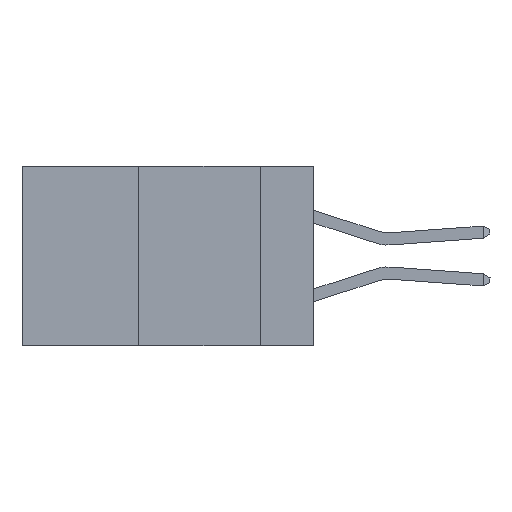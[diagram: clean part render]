
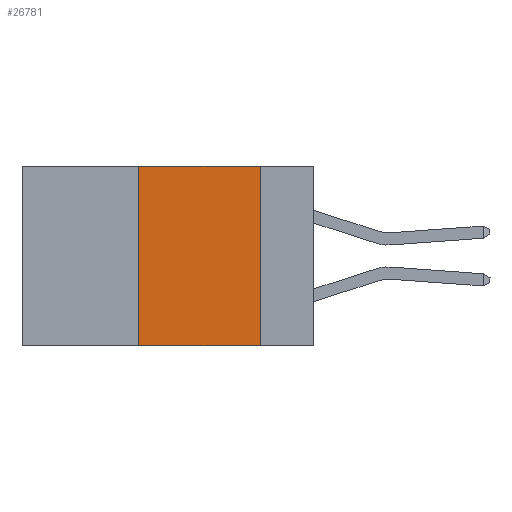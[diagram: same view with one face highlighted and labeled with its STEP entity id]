
A CAD part, left-side view. The second image highlights one B-rep face of the part: STEP entity #26781.
In plain terms, the highlighted planar face has unit normal (-1, 0, 0).
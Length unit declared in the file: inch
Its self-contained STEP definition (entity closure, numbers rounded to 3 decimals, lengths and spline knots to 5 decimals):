
#145 = VECTOR ( 'NONE', #16455, 39.37008 ) ;
#1751 = CARTESIAN_POINT ( 'NONE',  ( 0., 0.36, -0.37 ) ) ;
#2074 = VERTEX_POINT ( 'NONE', #1751 ) ;
#3510 = FACE_OUTER_BOUND ( 'NONE', #15893, .T. ) ;
#3734 = DIRECTION ( 'NONE',  ( 0., 0., -1. ) ) ;
#4413 = EDGE_CURVE ( 'NONE', #29092, #7162, #7078, .T. ) ;
#6048 = DIRECTION ( 'NONE',  ( 1., 0., 0. ) ) ;
#7078 = LINE ( 'NONE', #27547, #10424 ) ;
#7162 = VERTEX_POINT ( 'NONE', #16874 ) ;
#8538 = LINE ( 'NONE', #21929, #25552 ) ;
#8744 = DIRECTION ( 'NONE',  ( 0., -1., 0. ) ) ;
#10324 = VERTEX_POINT ( 'NONE', #17362 ) ;
#10424 = VECTOR ( 'NONE', #8744, 39.37008 ) ;
#11945 = ORIENTED_EDGE ( 'NONE', *, *, #4413, .F. ) ;
#13051 = LINE ( 'NONE', #28560, #13486 ) ;
#13486 = VECTOR ( 'NONE', #3734, 39.37008 ) ;
#14346 = EDGE_CURVE ( 'NONE', #2074, #29092, #23519, .T. ) ;
#15893 = EDGE_LOOP ( 'NONE', ( #25115, #11945, #27279, #17183 ) ) ;
#16455 = DIRECTION ( 'NONE',  ( 0., 0., 1. ) ) ;
#16599 = CARTESIAN_POINT ( 'NONE',  ( 0., 0.36, 0. ) ) ;
#16874 = CARTESIAN_POINT ( 'NONE',  ( 0., 0.11, 0. ) ) ;
#17183 = ORIENTED_EDGE ( 'NONE', *, *, #24644, .T. ) ;
#17362 = CARTESIAN_POINT ( 'NONE',  ( 0., 0.11, -0.37 ) ) ;
#19886 = PLANE ( 'NONE',  #23241 ) ;
#20110 = CARTESIAN_POINT ( 'NONE',  ( 0., 0.36, 0. ) ) ;
#21929 = CARTESIAN_POINT ( 'NONE',  ( 0., 0.6, -0.37 ) ) ;
#23241 = AXIS2_PLACEMENT_3D ( 'NONE', #26656, #6048, #28475 ) ;
#23264 = EDGE_CURVE ( 'NONE', #7162, #10324, #13051, .T. ) ;
#23519 = LINE ( 'NONE', #16599, #145 ) ;
#24638 = DIRECTION ( 'NONE',  ( 0., -1., 0. ) ) ;
#24644 = EDGE_CURVE ( 'NONE', #2074, #10324, #8538, .T. ) ;
#25115 = ORIENTED_EDGE ( 'NONE', *, *, #23264, .F. ) ;
#25552 = VECTOR ( 'NONE', #24638, 39.37008 ) ;
#26656 = CARTESIAN_POINT ( 'NONE',  ( 0., 0.6, 0. ) ) ;
#26781 = ADVANCED_FACE ( 'NONE', ( #3510 ), #19886, .F. ) ;
#27279 = ORIENTED_EDGE ( 'NONE', *, *, #14346, .F. ) ;
#27547 = CARTESIAN_POINT ( 'NONE',  ( 0., 0.6, 0. ) ) ;
#28475 = DIRECTION ( 'NONE',  ( 0., 0., -1. ) ) ;
#28560 = CARTESIAN_POINT ( 'NONE',  ( 0., 0.11, 0. ) ) ;
#29092 = VERTEX_POINT ( 'NONE', #20110 ) ;
